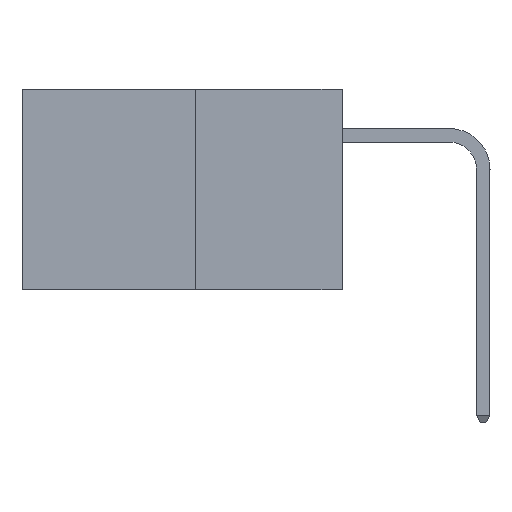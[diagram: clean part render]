
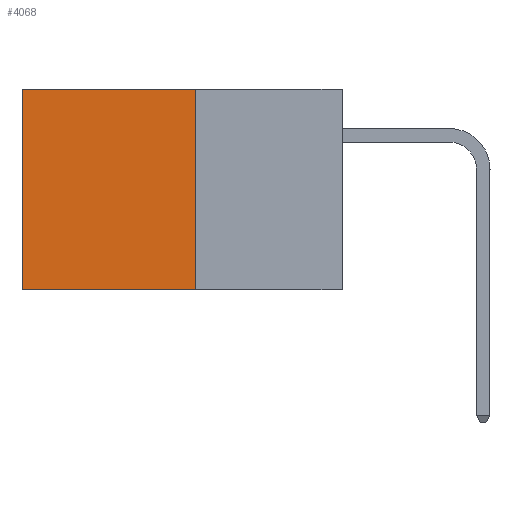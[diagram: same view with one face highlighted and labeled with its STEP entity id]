
A CAD part, left-side view. The second image highlights one B-rep face of the part: STEP entity #4068.
In plain terms, the highlighted planar face has unit normal (-1, 0, 0).
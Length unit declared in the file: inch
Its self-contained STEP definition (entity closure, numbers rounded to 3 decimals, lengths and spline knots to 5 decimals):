
#57 = VERTEX_POINT ( 'NONE', #12170 ) ;
#697 = EDGE_LOOP ( 'NONE', ( #10146, #3813, #7014, #4944 ) ) ;
#915 = LINE ( 'NONE', #6138, #10310 ) ;
#1310 = VERTEX_POINT ( 'NONE', #7296 ) ;
#1740 = EDGE_CURVE ( 'NONE', #1310, #12717, #8860, .T. ) ;
#1799 = CARTESIAN_POINT ( 'NONE',  ( 0.277, 0.59, -0.37 ) ) ;
#2267 = DIRECTION ( 'NONE',  ( 0., 0., -1. ) ) ;
#2980 = EDGE_CURVE ( 'NONE', #1310, #57, #915, .T. ) ;
#3545 = CARTESIAN_POINT ( 'NONE',  ( 0.277, 0.59, -0.37 ) ) ;
#3643 = VECTOR ( 'NONE', #2267, 39.37008 ) ;
#3813 = ORIENTED_EDGE ( 'NONE', *, *, #14684, .F. ) ;
#4068 = ADVANCED_FACE ( 'NONE', ( #10456 ), #8622, .F. ) ;
#4288 = CARTESIAN_POINT ( 'NONE',  ( 0.277, 0.27, -0.37 ) ) ;
#4944 = ORIENTED_EDGE ( 'NONE', *, *, #1740, .T. ) ;
#6138 = CARTESIAN_POINT ( 'NONE',  ( 0.277, 0.27, -0.37 ) ) ;
#6151 = DIRECTION ( 'NONE',  ( 0., 0., -1. ) ) ;
#6316 = LINE ( 'NONE', #4288, #15492 ) ;
#6846 = LINE ( 'NONE', #3545, #3643 ) ;
#6863 = EDGE_CURVE ( 'NONE', #12717, #13904, #6846, .T. ) ;
#7014 = ORIENTED_EDGE ( 'NONE', *, *, #2980, .F. ) ;
#7296 = CARTESIAN_POINT ( 'NONE',  ( 0.277, 0.27, 0. ) ) ;
#7882 = DIRECTION ( 'NONE',  ( 0., 1., 0. ) ) ;
#8046 = DIRECTION ( 'NONE',  ( 0., 1., 0. ) ) ;
#8487 = DIRECTION ( 'NONE',  ( 0., 0., -1. ) ) ;
#8488 = CARTESIAN_POINT ( 'NONE',  ( 0.277, 0.27, 0. ) ) ;
#8578 = DIRECTION ( 'NONE',  ( 1., 0., 0. ) ) ;
#8622 = PLANE ( 'NONE',  #10525 ) ;
#8835 = CARTESIAN_POINT ( 'NONE',  ( 0.277, 0.27, -0.37 ) ) ;
#8860 = LINE ( 'NONE', #8488, #11623 ) ;
#10146 = ORIENTED_EDGE ( 'NONE', *, *, #6863, .T. ) ;
#10310 = VECTOR ( 'NONE', #6151, 39.37008 ) ;
#10456 = FACE_OUTER_BOUND ( 'NONE', #697, .T. ) ;
#10525 = AXIS2_PLACEMENT_3D ( 'NONE', #8835, #8578, #8487 ) ;
#11623 = VECTOR ( 'NONE', #8046, 39.37008 ) ;
#12170 = CARTESIAN_POINT ( 'NONE',  ( 0.277, 0.27, -0.37 ) ) ;
#12717 = VERTEX_POINT ( 'NONE', #12744 ) ;
#12744 = CARTESIAN_POINT ( 'NONE',  ( 0.277, 0.59, 0. ) ) ;
#13904 = VERTEX_POINT ( 'NONE', #1799 ) ;
#14684 = EDGE_CURVE ( 'NONE', #57, #13904, #6316, .T. ) ;
#15492 = VECTOR ( 'NONE', #7882, 39.37008 ) ;
